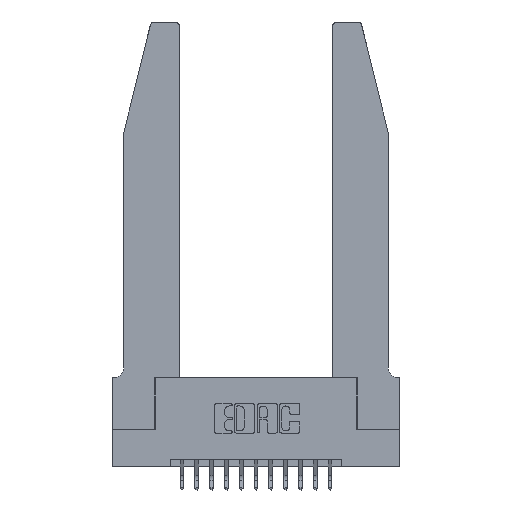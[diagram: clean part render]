
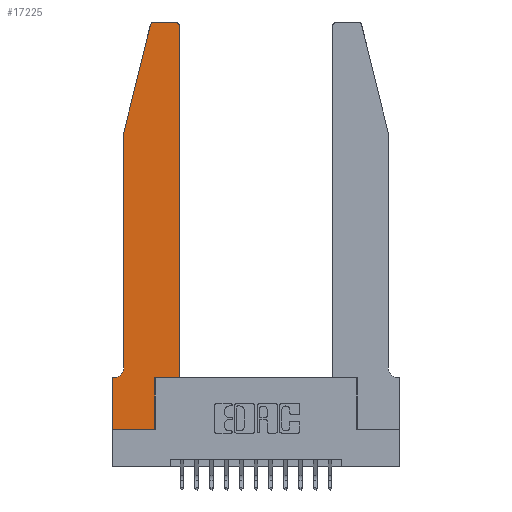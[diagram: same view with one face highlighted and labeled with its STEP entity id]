
A CAD part, top view. The second image highlights one B-rep face of the part: STEP entity #17225.
In plain terms, the highlighted planar face has unit normal (0, 0, 1).
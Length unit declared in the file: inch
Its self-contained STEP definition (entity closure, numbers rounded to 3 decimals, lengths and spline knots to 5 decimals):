
#189 = CIRCLE ( 'NONE', #1138, 0.03 ) ;
#511 = CARTESIAN_POINT ( 'NONE',  ( 0.4505, 0.35, 0.37 ) ) ;
#812 = DIRECTION ( 'NONE',  ( 1., 0., 0. ) ) ;
#1055 = DIRECTION ( 'NONE',  ( -0.239, -0.971, 0. ) ) ;
#1087 = CARTESIAN_POINT ( 'NONE',  ( 0., 0., 0.37 ) ) ;
#1138 = AXIS2_PLACEMENT_3D ( 'NONE', #7718, #15968, #17285 ) ;
#1399 = VECTOR ( 'NONE', #1055, 39.37008 ) ;
#1719 = DIRECTION ( 'NONE',  ( 1., 0., 0. ) ) ;
#1989 = CARTESIAN_POINT ( 'NONE',  ( 0.0755, 0.42, 0.37 ) ) ;
#2064 = VERTEX_POINT ( 'NONE', #2681 ) ;
#2071 = EDGE_CURVE ( 'NONE', #5228, #17515, #9311, .T. ) ;
#2681 = CARTESIAN_POINT ( 'NONE',  ( 0.2865, 0.35, 0.37 ) ) ;
#3553 = ORIENTED_EDGE ( 'NONE', *, *, #13795, .T. ) ;
#3645 = VERTEX_POINT ( 'NONE', #1989 ) ;
#4140 = DIRECTION ( 'NONE',  ( 1., 0., 0. ) ) ;
#4191 = DIRECTION ( 'NONE',  ( 0., -1., 0. ) ) ;
#4247 = CARTESIAN_POINT ( 'NONE',  ( 0.2605, 2.75, 0.37 ) ) ;
#4253 = CARTESIAN_POINT ( 'NONE',  ( 0.0755, 2., 0.37 ) ) ;
#4459 = FACE_OUTER_BOUND ( 'NONE', #15290, .T. ) ;
#4575 = EDGE_CURVE ( 'NONE', #9714, #4810, #7518, .T. ) ;
#4685 = VERTEX_POINT ( 'NONE', #6475 ) ;
#4810 = VERTEX_POINT ( 'NONE', #7062 ) ;
#4919 = LINE ( 'NONE', #1087, #11811 ) ;
#4946 = DIRECTION ( 'NONE',  ( -1., 0., 0. ) ) ;
#5116 = EDGE_CURVE ( 'NONE', #4810, #4685, #6617, .T. ) ;
#5228 = VERTEX_POINT ( 'NONE', #13574 ) ;
#5335 = ORIENTED_EDGE ( 'NONE', *, *, #14519, .T. ) ;
#5779 = ORIENTED_EDGE ( 'NONE', *, *, #12677, .T. ) ;
#6060 = CIRCLE ( 'NONE', #8941, 0.07 ) ;
#6475 = CARTESIAN_POINT ( 'NONE',  ( 0., 0., 0.37 ) ) ;
#6598 = ORIENTED_EDGE ( 'NONE', *, *, #4575, .T. ) ;
#6617 = LINE ( 'NONE', #13501, #14123 ) ;
#7062 = CARTESIAN_POINT ( 'NONE',  ( 0., 0.35, 0.37 ) ) ;
#7415 = LINE ( 'NONE', #4253, #9997 ) ;
#7518 = LINE ( 'NONE', #15566, #17778 ) ;
#7657 = CARTESIAN_POINT ( 'NONE',  ( 0.4205, 2.72, 0.37 ) ) ;
#7718 = CARTESIAN_POINT ( 'NONE',  ( 0.284, 2.72, 0.37 ) ) ;
#7769 = DIRECTION ( 'NONE',  ( 0., 0., 1. ) ) ;
#7957 = DIRECTION ( 'NONE',  ( 0., 1., 0. ) ) ;
#7978 = DIRECTION ( 'NONE',  ( 1., 0., 0. ) ) ;
#8378 = PLANE ( 'NONE',  #15468 ) ;
#8429 = EDGE_CURVE ( 'NONE', #3645, #9714, #6060, .T. ) ;
#8768 = DIRECTION ( 'NONE',  ( -1., 0., 0. ) ) ;
#8824 = DIRECTION ( 'NONE',  ( 0., 0., -1. ) ) ;
#8941 = AXIS2_PLACEMENT_3D ( 'NONE', #8944, #8824, #8768 ) ;
#8944 = CARTESIAN_POINT ( 'NONE',  ( 0.0055, 0.42, 0.37 ) ) ;
#9311 = LINE ( 'NONE', #4247, #12491 ) ;
#9446 = LINE ( 'NONE', #10755, #12204 ) ;
#9618 = AXIS2_PLACEMENT_3D ( 'NONE', #7657, #7769, #812 ) ;
#9714 = VERTEX_POINT ( 'NONE', #15867 ) ;
#9869 = LINE ( 'NONE', #13810, #16684 ) ;
#9997 = VECTOR ( 'NONE', #4191, 39.37008 ) ;
#10023 = ORIENTED_EDGE ( 'NONE', *, *, #17549, .T. ) ;
#10061 = ORIENTED_EDGE ( 'NONE', *, *, #12048, .T. ) ;
#10137 = EDGE_CURVE ( 'NONE', #14608, #3645, #7415, .T. ) ;
#10755 = CARTESIAN_POINT ( 'NONE',  ( 0.2865, 0.35, 0.37 ) ) ;
#10774 = DIRECTION ( 'NONE',  ( 0., -1., 0. ) ) ;
#11029 = CARTESIAN_POINT ( 'NONE',  ( 0., 0.35, 0.37 ) ) ;
#11333 = CARTESIAN_POINT ( 'NONE',  ( 0.4505, 2.72, 0.37 ) ) ;
#11675 = ORIENTED_EDGE ( 'NONE', *, *, #5116, .T. ) ;
#11811 = VECTOR ( 'NONE', #7978, 39.37008 ) ;
#11861 = VERTEX_POINT ( 'NONE', #11333 ) ;
#11986 = VECTOR ( 'NONE', #1719, 39.37008 ) ;
#12019 = CARTESIAN_POINT ( 'NONE',  ( 0.0755, 2., 0.37 ) ) ;
#12048 = EDGE_CURVE ( 'NONE', #17515, #15666, #189, .T. ) ;
#12204 = VECTOR ( 'NONE', #17722, 39.37008 ) ;
#12386 = DIRECTION ( 'NONE',  ( 0., 0., 1. ) ) ;
#12491 = VECTOR ( 'NONE', #16618, 39.37008 ) ;
#12569 = VERTEX_POINT ( 'NONE', #511 ) ;
#12592 = CIRCLE ( 'NONE', #9618, 0.03 ) ;
#12638 = VERTEX_POINT ( 'NONE', #14575 ) ;
#12677 = EDGE_CURVE ( 'NONE', #4685, #12638, #4919, .T. ) ;
#12929 = ORIENTED_EDGE ( 'NONE', *, *, #8429, .T. ) ;
#13248 = LINE ( 'NONE', #12019, #1399 ) ;
#13501 = CARTESIAN_POINT ( 'NONE',  ( 0., 0., 0.37 ) ) ;
#13574 = CARTESIAN_POINT ( 'NONE',  ( 0.4205, 2.75, 0.37 ) ) ;
#13795 = EDGE_CURVE ( 'NONE', #12638, #2064, #9446, .T. ) ;
#13810 = CARTESIAN_POINT ( 'NONE',  ( 0.4505, 0.35, 0.37 ) ) ;
#14100 = EDGE_CURVE ( 'NONE', #12569, #11861, #9869, .T. ) ;
#14109 = CARTESIAN_POINT ( 'NONE',  ( 0.4505, 0.35, 0.37 ) ) ;
#14123 = VECTOR ( 'NONE', #10774, 39.37008 ) ;
#14519 = EDGE_CURVE ( 'NONE', #11861, #5228, #12592, .T. ) ;
#14575 = CARTESIAN_POINT ( 'NONE',  ( 0.2865, 0., 0.37 ) ) ;
#14608 = VERTEX_POINT ( 'NONE', #14870 ) ;
#14690 = ORIENTED_EDGE ( 'NONE', *, *, #16243, .T. ) ;
#14870 = CARTESIAN_POINT ( 'NONE',  ( 0.0755, 2., 0.37 ) ) ;
#15073 = LINE ( 'NONE', #14109, #11986 ) ;
#15290 = EDGE_LOOP ( 'NONE', ( #16444, #10061, #10023, #17116, #12929, #6598, #11675, #5779, #3553, #14690, #16014, #5335 ) ) ;
#15455 = CARTESIAN_POINT ( 'NONE',  ( 0.25487, 2.72718, 0.37 ) ) ;
#15468 = AXIS2_PLACEMENT_3D ( 'NONE', #11029, #12386, #4140 ) ;
#15566 = CARTESIAN_POINT ( 'NONE',  ( 0.0755, 0.35, 0.37 ) ) ;
#15666 = VERTEX_POINT ( 'NONE', #15455 ) ;
#15867 = CARTESIAN_POINT ( 'NONE',  ( 0.0055, 0.35, 0.37 ) ) ;
#15968 = DIRECTION ( 'NONE',  ( 0., 0., 1. ) ) ;
#16014 = ORIENTED_EDGE ( 'NONE', *, *, #14100, .T. ) ;
#16147 = CARTESIAN_POINT ( 'NONE',  ( 0.284, 2.75, 0.37 ) ) ;
#16243 = EDGE_CURVE ( 'NONE', #2064, #12569, #15073, .T. ) ;
#16444 = ORIENTED_EDGE ( 'NONE', *, *, #2071, .T. ) ;
#16618 = DIRECTION ( 'NONE',  ( -1., 0., 0. ) ) ;
#16684 = VECTOR ( 'NONE', #7957, 39.37008 ) ;
#17116 = ORIENTED_EDGE ( 'NONE', *, *, #10137, .T. ) ;
#17225 = ADVANCED_FACE ( 'NONE', ( #4459 ), #8378, .T. ) ;
#17285 = DIRECTION ( 'NONE',  ( 1., 0., 0. ) ) ;
#17515 = VERTEX_POINT ( 'NONE', #16147 ) ;
#17549 = EDGE_CURVE ( 'NONE', #15666, #14608, #13248, .T. ) ;
#17722 = DIRECTION ( 'NONE',  ( 0., 1., 0. ) ) ;
#17778 = VECTOR ( 'NONE', #4946, 39.37008 ) ;
